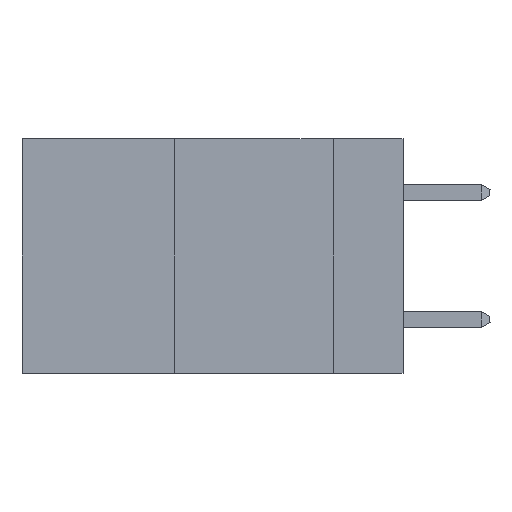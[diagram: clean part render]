
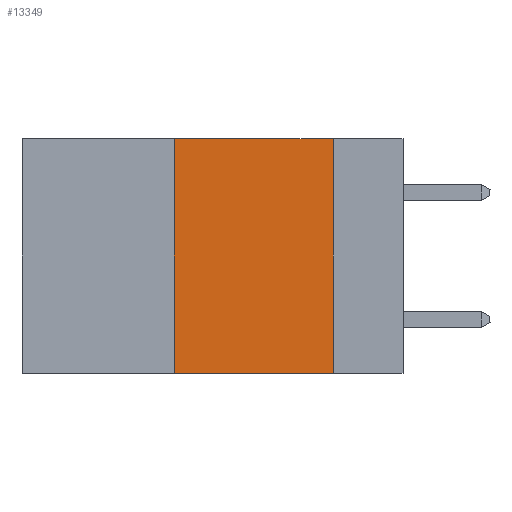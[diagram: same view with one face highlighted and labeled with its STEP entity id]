
A CAD part, left-side view. The second image highlights one B-rep face of the part: STEP entity #13349.
In plain terms, the highlighted planar face has unit normal (-1, 0, 0).
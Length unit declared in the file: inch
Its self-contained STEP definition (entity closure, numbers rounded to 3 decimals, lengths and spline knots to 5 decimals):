
#293 = PLANE ( 'NONE',  #26674 ) ;
#382 = DIRECTION ( 'NONE',  ( 0., 0., -1. ) ) ;
#679 = LINE ( 'NONE', #25440, #22782 ) ;
#833 = VECTOR ( 'NONE', #20251, 39.37008 ) ;
#1730 = VECTOR ( 'NONE', #14042, 39.37008 ) ;
#1894 = ORIENTED_EDGE ( 'NONE', *, *, #4992, .F. ) ;
#3508 = VERTEX_POINT ( 'NONE', #27154 ) ;
#3794 = DIRECTION ( 'NONE',  ( 0., -1., 0. ) ) ;
#4992 = EDGE_CURVE ( 'NONE', #3508, #24200, #15101, .T. ) ;
#6357 = LINE ( 'NONE', #26502, #1730 ) ;
#6604 = ORIENTED_EDGE ( 'NONE', *, *, #7765, .T. ) ;
#7765 = EDGE_CURVE ( 'NONE', #18747, #22147, #6357, .T. ) ;
#9471 = VECTOR ( 'NONE', #3794, 39.37008 ) ;
#12047 = EDGE_CURVE ( 'NONE', #18747, #3508, #14396, .T. ) ;
#12654 = FACE_OUTER_BOUND ( 'NONE', #20345, .T. ) ;
#13038 = ORIENTED_EDGE ( 'NONE', *, *, #15247, .F. ) ;
#13070 = CARTESIAN_POINT ( 'NONE',  ( 0., 0.11, 0. ) ) ;
#13349 = ADVANCED_FACE ( 'NONE', ( #12654 ), #293, .F. ) ;
#14042 = DIRECTION ( 'NONE',  ( 0., -1., 0. ) ) ;
#14232 = CARTESIAN_POINT ( 'NONE',  ( 0., 0.6, 0. ) ) ;
#14396 = LINE ( 'NONE', #25603, #833 ) ;
#15101 = LINE ( 'NONE', #14232, #9471 ) ;
#15247 = EDGE_CURVE ( 'NONE', #24200, #22147, #679, .T. ) ;
#17514 = CARTESIAN_POINT ( 'NONE',  ( 0., 0.6, 0. ) ) ;
#18747 = VERTEX_POINT ( 'NONE', #24291 ) ;
#19689 = CARTESIAN_POINT ( 'NONE',  ( 0., 0.11, -0.37 ) ) ;
#20251 = DIRECTION ( 'NONE',  ( 0., 0., 1. ) ) ;
#20345 = EDGE_LOOP ( 'NONE', ( #13038, #1894, #20496, #6604 ) ) ;
#20496 = ORIENTED_EDGE ( 'NONE', *, *, #12047, .F. ) ;
#21752 = DIRECTION ( 'NONE',  ( 1., 0., 0. ) ) ;
#22147 = VERTEX_POINT ( 'NONE', #19689 ) ;
#22782 = VECTOR ( 'NONE', #382, 39.37008 ) ;
#24200 = VERTEX_POINT ( 'NONE', #13070 ) ;
#24291 = CARTESIAN_POINT ( 'NONE',  ( 0., 0.36, -0.37 ) ) ;
#25440 = CARTESIAN_POINT ( 'NONE',  ( 0., 0.11, 0. ) ) ;
#25603 = CARTESIAN_POINT ( 'NONE',  ( 0., 0.36, 0. ) ) ;
#26083 = DIRECTION ( 'NONE',  ( 0., 0., -1. ) ) ;
#26502 = CARTESIAN_POINT ( 'NONE',  ( 0., 0.6, -0.37 ) ) ;
#26674 = AXIS2_PLACEMENT_3D ( 'NONE', #17514, #21752, #26083 ) ;
#27154 = CARTESIAN_POINT ( 'NONE',  ( 0., 0.36, 0. ) ) ;
